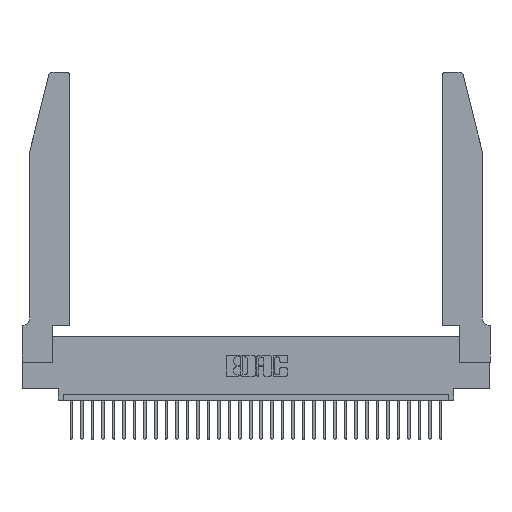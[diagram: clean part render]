
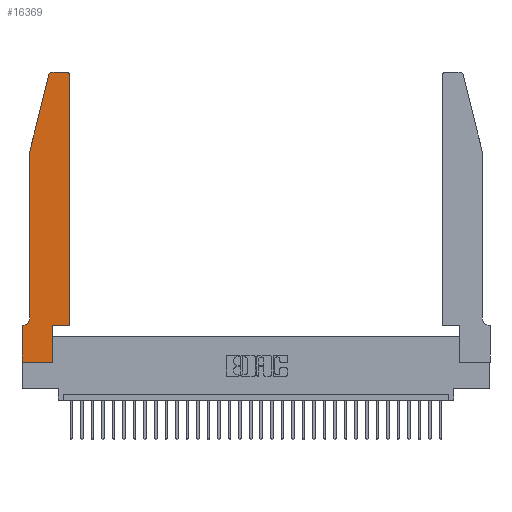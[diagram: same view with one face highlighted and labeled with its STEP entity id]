
A CAD part, top view. The second image highlights one B-rep face of the part: STEP entity #16369.
In plain terms, the highlighted planar face has unit normal (0, 0, 1).
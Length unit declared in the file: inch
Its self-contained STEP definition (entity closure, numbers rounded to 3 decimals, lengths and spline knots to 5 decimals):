
#186 = EDGE_CURVE ( 'NONE', #25050, #29941, #17824, .T. ) ;
#962 = CARTESIAN_POINT ( 'NONE',  ( 0.2865, 0., 0.37 ) ) ;
#1086 = EDGE_LOOP ( 'NONE', ( #18335, #10824, #22710, #4607, #7169, #24500, #6250, #1299, #1577, #30306, #29300, #14417 ) ) ;
#1299 = ORIENTED_EDGE ( 'NONE', *, *, #3362, .T. ) ;
#1577 = ORIENTED_EDGE ( 'NONE', *, *, #11082, .T. ) ;
#2714 = EDGE_CURVE ( 'NONE', #29941, #26696, #26621, .T. ) ;
#2941 = CARTESIAN_POINT ( 'NONE',  ( 0.284, 2.75, 0.37 ) ) ;
#3035 = DIRECTION ( 'NONE',  ( 0., 0., -1. ) ) ;
#3362 = EDGE_CURVE ( 'NONE', #14507, #10258, #25432, .T. ) ;
#3510 = AXIS2_PLACEMENT_3D ( 'NONE', #12980, #3035, #15572 ) ;
#3597 = VECTOR ( 'NONE', #25718, 39.37008 ) ;
#3718 = DIRECTION ( 'NONE',  ( 1., 0., 0. ) ) ;
#4592 = EDGE_CURVE ( 'NONE', #5265, #29613, #31327, .T. ) ;
#4607 = ORIENTED_EDGE ( 'NONE', *, *, #15273, .T. ) ;
#4652 = DIRECTION ( 'NONE',  ( -1., 0., 0. ) ) ;
#5126 = AXIS2_PLACEMENT_3D ( 'NONE', #9784, #18020, #5812 ) ;
#5265 = VERTEX_POINT ( 'NONE', #7772 ) ;
#5463 = LINE ( 'NONE', #6477, #28036 ) ;
#5473 = CARTESIAN_POINT ( 'NONE',  ( 0.2865, 0.35, 0.37 ) ) ;
#5498 = FACE_OUTER_BOUND ( 'NONE', #1086, .T. ) ;
#5600 = CARTESIAN_POINT ( 'NONE',  ( 0.2605, 2.75, 0.37 ) ) ;
#5765 = CARTESIAN_POINT ( 'NONE',  ( 0.0055, 0.35, 0.37 ) ) ;
#5812 = DIRECTION ( 'NONE',  ( 1., 0., 0. ) ) ;
#6250 = ORIENTED_EDGE ( 'NONE', *, *, #30049, .T. ) ;
#6477 = CARTESIAN_POINT ( 'NONE',  ( 0.4505, 0.35, 0.37 ) ) ;
#6596 = VERTEX_POINT ( 'NONE', #7806 ) ;
#7104 = CARTESIAN_POINT ( 'NONE',  ( 0.0755, 2., 0.37 ) ) ;
#7169 = ORIENTED_EDGE ( 'NONE', *, *, #186, .T. ) ;
#7772 = CARTESIAN_POINT ( 'NONE',  ( 0.4505, 0.35, 0.37 ) ) ;
#7806 = CARTESIAN_POINT ( 'NONE',  ( 0.25487, 2.72718, 0.37 ) ) ;
#7890 = AXIS2_PLACEMENT_3D ( 'NONE', #27331, #14503, #16991 ) ;
#8299 = VECTOR ( 'NONE', #26373, 39.37008 ) ;
#9784 = CARTESIAN_POINT ( 'NONE',  ( 0.4205, 2.72, 0.37 ) ) ;
#10038 = CARTESIAN_POINT ( 'NONE',  ( 0., 0., 0.37 ) ) ;
#10258 = VERTEX_POINT ( 'NONE', #962 ) ;
#10601 = CARTESIAN_POINT ( 'NONE',  ( 0.0755, 2., 0.37 ) ) ;
#10824 = ORIENTED_EDGE ( 'NONE', *, *, #12498, .T. ) ;
#11082 = EDGE_CURVE ( 'NONE', #10258, #18463, #32457, .T. ) ;
#11766 = DIRECTION ( 'NONE',  ( 0., 0., 1. ) ) ;
#11823 = PLANE ( 'NONE',  #7890 ) ;
#11971 = VECTOR ( 'NONE', #26183, 39.37008 ) ;
#12006 = VECTOR ( 'NONE', #31567, 39.37008 ) ;
#12498 = EDGE_CURVE ( 'NONE', #14125, #6596, #31585, .T. ) ;
#12980 = CARTESIAN_POINT ( 'NONE',  ( 0.0055, 0.42, 0.37 ) ) ;
#14125 = VERTEX_POINT ( 'NONE', #2941 ) ;
#14276 = VECTOR ( 'NONE', #29682, 39.37008 ) ;
#14329 = VECTOR ( 'NONE', #4652, 39.37008 ) ;
#14417 = ORIENTED_EDGE ( 'NONE', *, *, #25452, .T. ) ;
#14503 = DIRECTION ( 'NONE',  ( 0., 0., 1. ) ) ;
#14507 = VERTEX_POINT ( 'NONE', #10038 ) ;
#14863 = VERTEX_POINT ( 'NONE', #10601 ) ;
#15273 = EDGE_CURVE ( 'NONE', #14863, #25050, #18271, .T. ) ;
#15572 = DIRECTION ( 'NONE',  ( -1., 0., 0. ) ) ;
#15680 = CARTESIAN_POINT ( 'NONE',  ( 0.0755, 2., 0.37 ) ) ;
#15697 = EDGE_CURVE ( 'NONE', #25834, #14125, #27723, .T. ) ;
#16369 = ADVANCED_FACE ( 'NONE', ( #5498 ), #11823, .T. ) ;
#16385 = AXIS2_PLACEMENT_3D ( 'NONE', #26954, #11766, #24512 ) ;
#16991 = DIRECTION ( 'NONE',  ( 1., 0., 0. ) ) ;
#17824 = CIRCLE ( 'NONE', #3510, 0.07 ) ;
#17847 = EDGE_CURVE ( 'NONE', #6596, #14863, #23980, .T. ) ;
#17865 = VECTOR ( 'NONE', #26061, 39.37008 ) ;
#18020 = DIRECTION ( 'NONE',  ( 0., 0., 1. ) ) ;
#18271 = LINE ( 'NONE', #15680, #3597 ) ;
#18335 = ORIENTED_EDGE ( 'NONE', *, *, #15697, .T. ) ;
#18463 = VERTEX_POINT ( 'NONE', #29718 ) ;
#18895 = VECTOR ( 'NONE', #27342, 39.37008 ) ;
#19245 = CARTESIAN_POINT ( 'NONE',  ( 0.4505, 2.72, 0.37 ) ) ;
#19851 = CARTESIAN_POINT ( 'NONE',  ( 0.0755, 0.35, 0.37 ) ) ;
#19933 = EDGE_CURVE ( 'NONE', #18463, #5265, #5463, .T. ) ;
#21496 = CARTESIAN_POINT ( 'NONE',  ( 0., 0.35, 0.37 ) ) ;
#21582 = LINE ( 'NONE', #26784, #12006 ) ;
#22076 = CARTESIAN_POINT ( 'NONE',  ( 0.4505, 0.35, 0.37 ) ) ;
#22710 = ORIENTED_EDGE ( 'NONE', *, *, #17847, .T. ) ;
#23980 = LINE ( 'NONE', #7104, #18895 ) ;
#24500 = ORIENTED_EDGE ( 'NONE', *, *, #2714, .T. ) ;
#24512 = DIRECTION ( 'NONE',  ( 1., 0., 0. ) ) ;
#25050 = VERTEX_POINT ( 'NONE', #25310 ) ;
#25310 = CARTESIAN_POINT ( 'NONE',  ( 0.0755, 0.42, 0.37 ) ) ;
#25432 = LINE ( 'NONE', #26068, #11971 ) ;
#25452 = EDGE_CURVE ( 'NONE', #29613, #25834, #28897, .T. ) ;
#25604 = CARTESIAN_POINT ( 'NONE',  ( 0.4205, 2.75, 0.37 ) ) ;
#25718 = DIRECTION ( 'NONE',  ( 0., -1., 0. ) ) ;
#25834 = VERTEX_POINT ( 'NONE', #25604 ) ;
#26061 = DIRECTION ( 'NONE',  ( -1., 0., 0. ) ) ;
#26068 = CARTESIAN_POINT ( 'NONE',  ( 0., 0., 0.37 ) ) ;
#26183 = DIRECTION ( 'NONE',  ( 1., 0., 0. ) ) ;
#26373 = DIRECTION ( 'NONE',  ( 0., 1., 0. ) ) ;
#26621 = LINE ( 'NONE', #19851, #14329 ) ;
#26696 = VERTEX_POINT ( 'NONE', #21496 ) ;
#26784 = CARTESIAN_POINT ( 'NONE',  ( 0., 0., 0.37 ) ) ;
#26954 = CARTESIAN_POINT ( 'NONE',  ( 0.284, 2.72, 0.37 ) ) ;
#27331 = CARTESIAN_POINT ( 'NONE',  ( 0., 0.35, 0.37 ) ) ;
#27342 = DIRECTION ( 'NONE',  ( -0.239, -0.971, 0. ) ) ;
#27723 = LINE ( 'NONE', #5600, #17865 ) ;
#28036 = VECTOR ( 'NONE', #3718, 39.37008 ) ;
#28897 = CIRCLE ( 'NONE', #5126, 0.03 ) ;
#29300 = ORIENTED_EDGE ( 'NONE', *, *, #4592, .T. ) ;
#29613 = VERTEX_POINT ( 'NONE', #19245 ) ;
#29682 = DIRECTION ( 'NONE',  ( 0., 1., 0. ) ) ;
#29718 = CARTESIAN_POINT ( 'NONE',  ( 0.2865, 0.35, 0.37 ) ) ;
#29941 = VERTEX_POINT ( 'NONE', #5765 ) ;
#30049 = EDGE_CURVE ( 'NONE', #26696, #14507, #21582, .T. ) ;
#30306 = ORIENTED_EDGE ( 'NONE', *, *, #19933, .T. ) ;
#31327 = LINE ( 'NONE', #22076, #14276 ) ;
#31567 = DIRECTION ( 'NONE',  ( 0., -1., 0. ) ) ;
#31585 = CIRCLE ( 'NONE', #16385, 0.03 ) ;
#32457 = LINE ( 'NONE', #5473, #8299 ) ;
